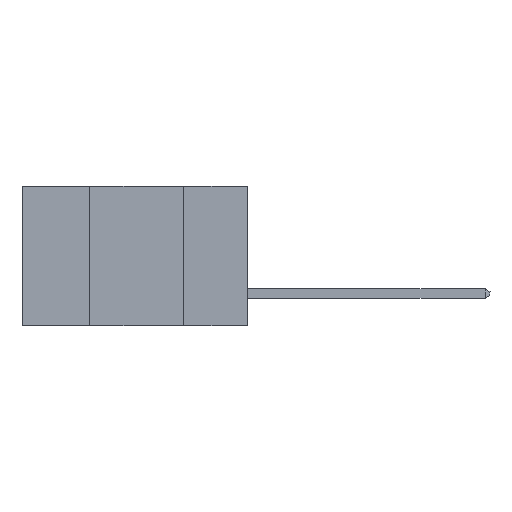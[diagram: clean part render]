
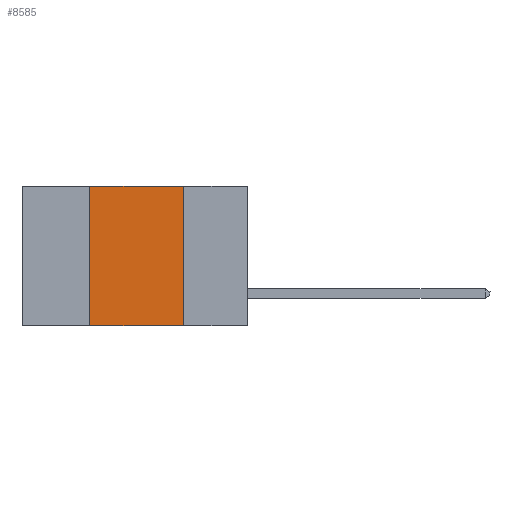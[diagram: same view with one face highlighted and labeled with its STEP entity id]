
A CAD part, left-side view. The second image highlights one B-rep face of the part: STEP entity #8585.
In plain terms, the highlighted planar face has unit normal (-1, 0, 0).
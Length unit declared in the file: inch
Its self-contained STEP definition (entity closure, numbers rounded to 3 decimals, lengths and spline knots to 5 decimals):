
#278 = EDGE_CURVE ( 'NONE', #3895, #2829, #5269, .T. ) ;
#660 = ORIENTED_EDGE ( 'NONE', *, *, #4274, .F. ) ;
#1120 = LINE ( 'NONE', #5823, #9299 ) ;
#1378 = VECTOR ( 'NONE', #8313, 39.37008 ) ;
#1386 = FACE_OUTER_BOUND ( 'NONE', #3148, .T. ) ;
#1611 = CARTESIAN_POINT ( 'NONE',  ( 0., 0.6, -0.37 ) ) ;
#2048 = CARTESIAN_POINT ( 'NONE',  ( 0., 0.17, -0.37 ) ) ;
#2196 = DIRECTION ( 'NONE',  ( 0., 0., 1. ) ) ;
#2301 = LINE ( 'NONE', #1611, #5284 ) ;
#2473 = CARTESIAN_POINT ( 'NONE',  ( 0., 0.17, 0. ) ) ;
#2829 = VERTEX_POINT ( 'NONE', #2473 ) ;
#3148 = EDGE_LOOP ( 'NONE', ( #660, #7668, #7502, #5251 ) ) ;
#3755 = PLANE ( 'NONE',  #7465 ) ;
#3895 = VERTEX_POINT ( 'NONE', #8693 ) ;
#4274 = EDGE_CURVE ( 'NONE', #2829, #8534, #6461, .T. ) ;
#4398 = EDGE_CURVE ( 'NONE', #5025, #3895, #1120, .T. ) ;
#5025 = VERTEX_POINT ( 'NONE', #7562 ) ;
#5060 = CARTESIAN_POINT ( 'NONE',  ( 0., 0.6, 0. ) ) ;
#5158 = DIRECTION ( 'NONE',  ( 1., 0., 0. ) ) ;
#5251 = ORIENTED_EDGE ( 'NONE', *, *, #9106, .T. ) ;
#5269 = LINE ( 'NONE', #7422, #1378 ) ;
#5284 = VECTOR ( 'NONE', #6076, 39.37008 ) ;
#5823 = CARTESIAN_POINT ( 'NONE',  ( 0., 0.42, -0.37 ) ) ;
#6076 = DIRECTION ( 'NONE',  ( 0., -1., 0. ) ) ;
#6461 = LINE ( 'NONE', #2048, #8373 ) ;
#6680 = DIRECTION ( 'NONE',  ( 0., 0., -1. ) ) ;
#7177 = CARTESIAN_POINT ( 'NONE',  ( 0., 0.17, -0.37 ) ) ;
#7422 = CARTESIAN_POINT ( 'NONE',  ( 0., 0.6, 0. ) ) ;
#7465 = AXIS2_PLACEMENT_3D ( 'NONE', #5060, #5158, #6680 ) ;
#7502 = ORIENTED_EDGE ( 'NONE', *, *, #4398, .F. ) ;
#7562 = CARTESIAN_POINT ( 'NONE',  ( 0., 0.42, -0.37 ) ) ;
#7668 = ORIENTED_EDGE ( 'NONE', *, *, #278, .F. ) ;
#8313 = DIRECTION ( 'NONE',  ( 0., -1., 0. ) ) ;
#8373 = VECTOR ( 'NONE', #9358, 39.37008 ) ;
#8534 = VERTEX_POINT ( 'NONE', #7177 ) ;
#8585 = ADVANCED_FACE ( 'NONE', ( #1386 ), #3755, .F. ) ;
#8693 = CARTESIAN_POINT ( 'NONE',  ( 0., 0.42, 0. ) ) ;
#9106 = EDGE_CURVE ( 'NONE', #5025, #8534, #2301, .T. ) ;
#9299 = VECTOR ( 'NONE', #2196, 39.37008 ) ;
#9358 = DIRECTION ( 'NONE',  ( 0., 0., -1. ) ) ;
